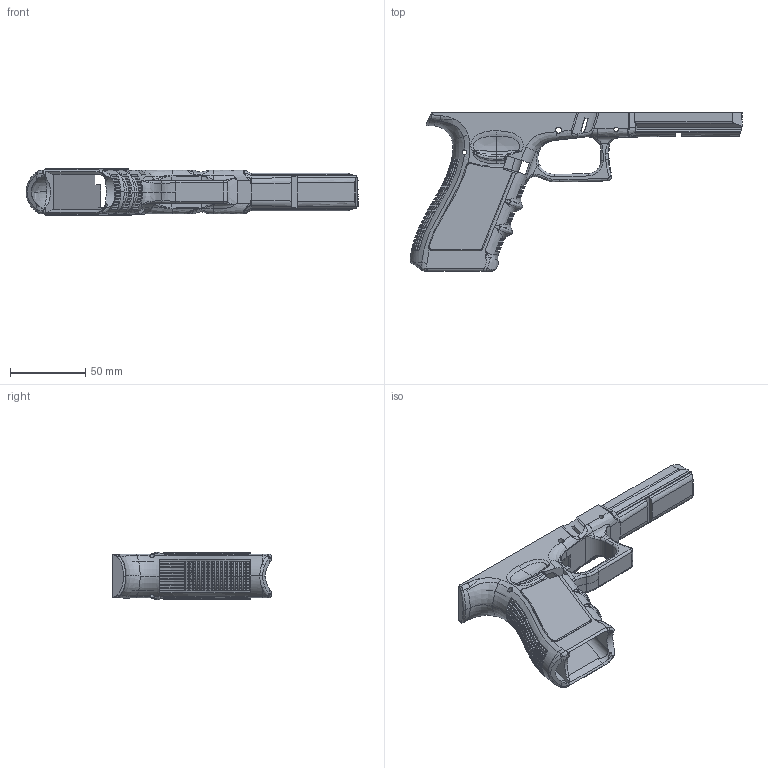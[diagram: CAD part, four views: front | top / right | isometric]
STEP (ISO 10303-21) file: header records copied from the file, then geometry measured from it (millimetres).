
FILE_DESCRIPTION(/* description */ (''),/* implementation_level */ '2;1');
FILE_NAME(/* name */ 'PY2A G34 LDC.step',/* time_stamp */ '2022-04-03T19:26:55-05:00',/* author */ (''),/* organization */ (''),/* preprocessor_version */ 'ST-DEVELOPER v18.1',/* originating_system */ 'Autodesk Translation Framework v10.14.0.1471',/* authorisation */ '');
FILE_SCHEMA (('AUTOMOTIVE_DESIGN { 1 0 10303 214 3 1 1 }'));
Products named in the file (3): PY2A G34 LDC Custom; PrintYour2A G17.8; Body
Assembly tree (2 placements, depth 3):
  PY2A G34 LDC Custom
    PrintYour2A G17.8
      Body
Bounding box: 220.76 x 105.56 x 31.87 mm (x, y, z)
Volume: 96167.4 mm3; surface area: 56055.1 mm2
Topology: 2 solids, 3 shells, 2050 faces, 5892 edges, 3826 vertices
Faces by surface type: bspline 879, plane 831, cylinder 314, torus 20, cone 4, sphere 2
Full cylindrical faces by diameter (mm): 1.933 x1, 3.05 x2, 3.146 x2, 4.1 x2
Entity records: 180994 total; most frequent: CARTESIAN_POINT 131746, ORIENTED_EDGE 11754, DIRECTION 8586, EDGE_CURVE 5877, VERTEX_POINT 3826, AXIS2_PLACEMENT_3D 3039, LINE 2508, VECTOR 2508
